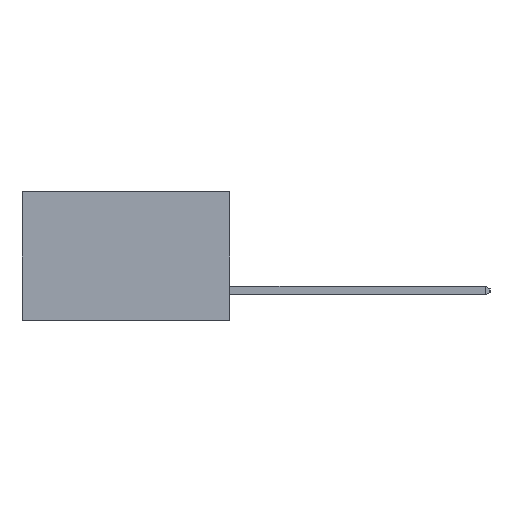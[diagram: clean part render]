
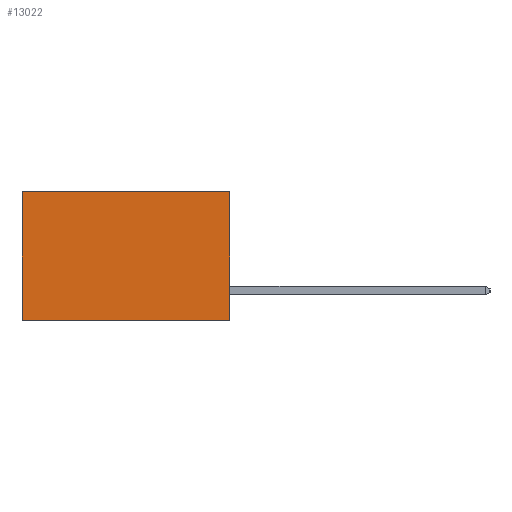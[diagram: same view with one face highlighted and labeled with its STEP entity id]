
A CAD part, left-side view. The second image highlights one B-rep face of the part: STEP entity #13022.
In plain terms, the highlighted planar face has unit normal (-1, 0, 0).
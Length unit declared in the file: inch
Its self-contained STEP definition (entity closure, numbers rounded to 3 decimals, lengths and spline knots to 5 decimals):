
#134 = DIRECTION ( 'NONE',  ( 0., 1., 0. ) ) ;
#168 = PLANE ( 'NONE',  #17744 ) ;
#226 = CARTESIAN_POINT ( 'NONE',  ( 0.2615, 0., 0. ) ) ;
#996 = FACE_OUTER_BOUND ( 'NONE', #16785, .T. ) ;
#2158 = DIRECTION ( 'NONE',  ( 0., 0., -1. ) ) ;
#2426 = LINE ( 'NONE', #226, #9893 ) ;
#2684 = LINE ( 'NONE', #9619, #17325 ) ;
#3198 = VERTEX_POINT ( 'NONE', #9410 ) ;
#3368 = VERTEX_POINT ( 'NONE', #17809 ) ;
#4317 = EDGE_CURVE ( 'NONE', #3198, #16717, #2426, .T. ) ;
#4875 = DIRECTION ( 'NONE',  ( 0., 0., -1. ) ) ;
#5072 = ORIENTED_EDGE ( 'NONE', *, *, #7878, .F. ) ;
#5458 = EDGE_CURVE ( 'NONE', #16717, #8296, #9623, .T. ) ;
#6308 = CARTESIAN_POINT ( 'NONE',  ( 0.2615, 0., -0.37 ) ) ;
#7803 = DIRECTION ( 'NONE',  ( 0., 0., -1. ) ) ;
#7878 = EDGE_CURVE ( 'NONE', #3368, #8296, #13176, .T. ) ;
#8296 = VERTEX_POINT ( 'NONE', #13656 ) ;
#8657 = ORIENTED_EDGE ( 'NONE', *, *, #13863, .F. ) ;
#9141 = VECTOR ( 'NONE', #4875, 39.37008 ) ;
#9410 = CARTESIAN_POINT ( 'NONE',  ( 0.2615, 0., 0. ) ) ;
#9619 = CARTESIAN_POINT ( 'NONE',  ( 0.2615, 0., -0.37 ) ) ;
#9623 = LINE ( 'NONE', #15425, #9141 ) ;
#9893 = VECTOR ( 'NONE', #134, 39.37008 ) ;
#11809 = VECTOR ( 'NONE', #16988, 39.37008 ) ;
#12089 = ORIENTED_EDGE ( 'NONE', *, *, #5458, .T. ) ;
#13022 = ADVANCED_FACE ( 'NONE', ( #996 ), #168, .F. ) ;
#13176 = LINE ( 'NONE', #17277, #11809 ) ;
#13656 = CARTESIAN_POINT ( 'NONE',  ( 0.2615, 0.6, -0.37 ) ) ;
#13703 = CARTESIAN_POINT ( 'NONE',  ( 0.2615, 0.6, 0. ) ) ;
#13863 = EDGE_CURVE ( 'NONE', #3198, #3368, #2684, .T. ) ;
#14411 = ORIENTED_EDGE ( 'NONE', *, *, #4317, .T. ) ;
#15425 = CARTESIAN_POINT ( 'NONE',  ( 0.2615, 0.6, -0.37 ) ) ;
#16441 = DIRECTION ( 'NONE',  ( 1., 0., 0. ) ) ;
#16717 = VERTEX_POINT ( 'NONE', #13703 ) ;
#16785 = EDGE_LOOP ( 'NONE', ( #12089, #5072, #8657, #14411 ) ) ;
#16988 = DIRECTION ( 'NONE',  ( 0., 1., 0. ) ) ;
#17277 = CARTESIAN_POINT ( 'NONE',  ( 0.2615, 0., -0.37 ) ) ;
#17325 = VECTOR ( 'NONE', #2158, 39.37008 ) ;
#17744 = AXIS2_PLACEMENT_3D ( 'NONE', #6308, #16441, #7803 ) ;
#17809 = CARTESIAN_POINT ( 'NONE',  ( 0.2615, 0., -0.37 ) ) ;
